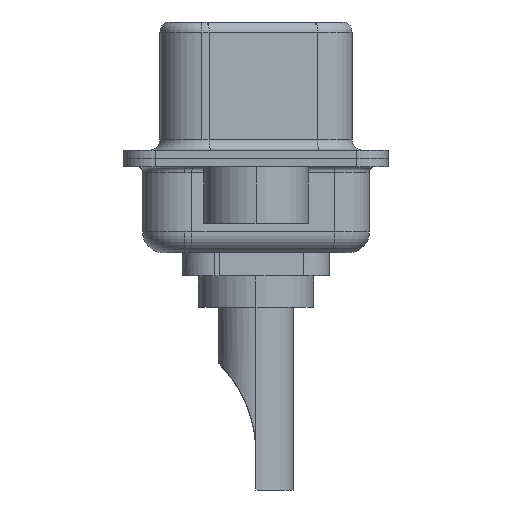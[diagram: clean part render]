
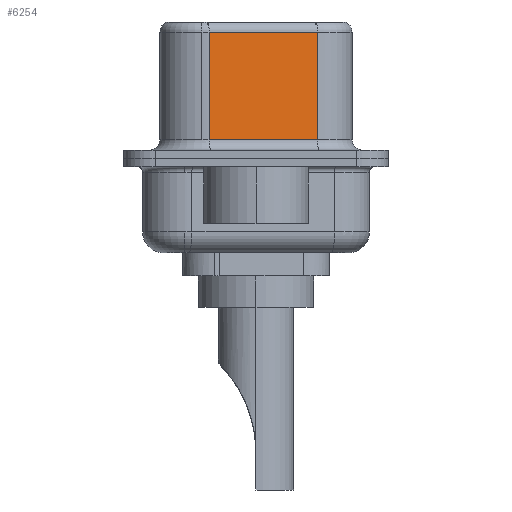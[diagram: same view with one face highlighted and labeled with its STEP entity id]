
A CAD part, left-side view. The second image highlights one B-rep face of the part: STEP entity #6254.
In plain terms, the highlighted planar face has unit normal (-0.985, -0.174, 0).
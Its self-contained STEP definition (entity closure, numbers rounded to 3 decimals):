
#256 = DIRECTION ( 'NONE',  ( 0.174, -0.985, 0. ) ) ;
#942 = ORIENTED_EDGE ( 'NONE', *, *, #12048, .T. ) ;
#1114 = VECTOR ( 'NONE', #7524, 1000. ) ;
#1563 = LINE ( 'NONE', #14904, #1114 ) ;
#1594 = VECTOR ( 'NONE', #256, 1000. ) ;
#2333 = VERTEX_POINT ( 'NONE', #11091 ) ;
#3888 = LINE ( 'NONE', #9012, #18363 ) ;
#4092 = EDGE_LOOP ( 'NONE', ( #11051, #942, #18366, #9014 ) ) ;
#4298 = VERTEX_POINT ( 'NONE', #6114 ) ;
#4375 = FACE_OUTER_BOUND ( 'NONE', #4092, .T. ) ;
#4665 = DIRECTION ( 'NONE',  ( -0.174, 0.985, 0. ) ) ;
#4724 = DIRECTION ( 'NONE',  ( 0.985, 0.174, 0. ) ) ;
#5729 = VECTOR ( 'NONE', #15026, 1000. ) ;
#5966 = CARTESIAN_POINT ( 'NONE',  ( 4.58, -2.927, 6.02 ) ) ;
#6114 = CARTESIAN_POINT ( 'NONE',  ( 3.67, 2.233, 6.02 ) ) ;
#6254 = ADVANCED_FACE ( 'NONE', ( #4375 ), #11568, .F. ) ;
#6549 = VERTEX_POINT ( 'NONE', #17348 ) ;
#7524 = DIRECTION ( 'NONE',  ( 0., 0., -1. ) ) ;
#8086 = AXIS2_PLACEMENT_3D ( 'NONE', #17923, #4724, #4665 ) ;
#9012 = CARTESIAN_POINT ( 'NONE',  ( 4.58, -2.927, 6.02 ) ) ;
#9014 = ORIENTED_EDGE ( 'NONE', *, *, #12144, .T. ) ;
#9197 = DIRECTION ( 'NONE',  ( -0.174, 0.985, 0. ) ) ;
#11051 = ORIENTED_EDGE ( 'NONE', *, *, #12465, .F. ) ;
#11091 = CARTESIAN_POINT ( 'NONE',  ( 4.58, -2.927, 0.9 ) ) ;
#11568 = PLANE ( 'NONE',  #8086 ) ;
#12048 = EDGE_CURVE ( 'NONE', #12882, #4298, #3888, .T. ) ;
#12144 = EDGE_CURVE ( 'NONE', #6549, #2333, #14665, .T. ) ;
#12465 = EDGE_CURVE ( 'NONE', #12882, #2333, #16249, .T. ) ;
#12882 = VERTEX_POINT ( 'NONE', #5966 ) ;
#13515 = EDGE_CURVE ( 'NONE', #4298, #6549, #1563, .T. ) ;
#14665 = LINE ( 'NONE', #16555, #1594 ) ;
#14904 = CARTESIAN_POINT ( 'NONE',  ( 3.67, 2.233, 6.52 ) ) ;
#15026 = DIRECTION ( 'NONE',  ( 0., 0., -1. ) ) ;
#16249 = LINE ( 'NONE', #18951, #5729 ) ;
#16555 = CARTESIAN_POINT ( 'NONE',  ( 4.58, -2.927, 0.9 ) ) ;
#17348 = CARTESIAN_POINT ( 'NONE',  ( 3.67, 2.233, 0.9 ) ) ;
#17923 = CARTESIAN_POINT ( 'NONE',  ( 4.58, -2.927, 6.52 ) ) ;
#18363 = VECTOR ( 'NONE', #9197, 1000. ) ;
#18366 = ORIENTED_EDGE ( 'NONE', *, *, #13515, .T. ) ;
#18951 = CARTESIAN_POINT ( 'NONE',  ( 4.58, -2.927, 6.52 ) ) ;
